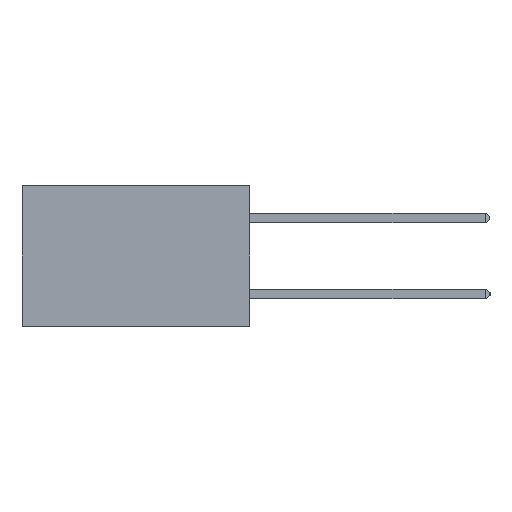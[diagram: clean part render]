
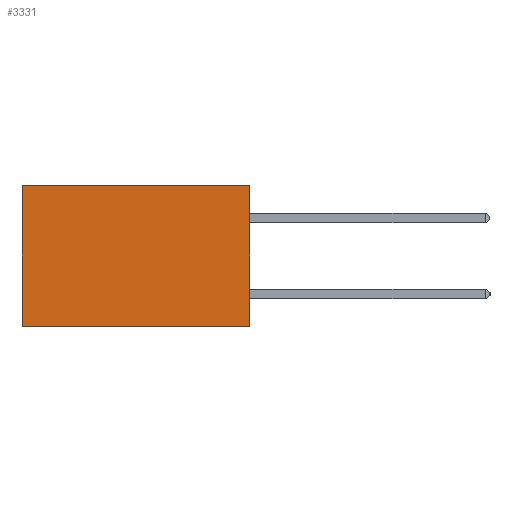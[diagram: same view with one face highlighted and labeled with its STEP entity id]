
A CAD part, left-side view. The second image highlights one B-rep face of the part: STEP entity #3331.
In plain terms, the highlighted planar face has unit normal (-1, 0, 0).
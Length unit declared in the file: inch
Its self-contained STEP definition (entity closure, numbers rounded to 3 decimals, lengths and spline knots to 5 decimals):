
#175 = VECTOR ( 'NONE', #521, 39.37008 ) ;
#521 = DIRECTION ( 'NONE',  ( 0., 1., 0. ) ) ;
#916 = EDGE_CURVE ( 'NONE', #8015, #15367, #3293, .T. ) ;
#978 = LINE ( 'NONE', #11055, #4941 ) ;
#2094 = CARTESIAN_POINT ( 'NONE',  ( 0.2875, 0., 0. ) ) ;
#3293 = LINE ( 'NONE', #18927, #20393 ) ;
#3331 = ADVANCED_FACE ( 'NONE', ( #19078 ), #16907, .F. ) ;
#3595 = EDGE_CURVE ( 'NONE', #15367, #18838, #9083, .T. ) ;
#4389 = DIRECTION ( 'NONE',  ( 0., 1., 0. ) ) ;
#4941 = VECTOR ( 'NONE', #12691, 39.37008 ) ;
#7116 = CARTESIAN_POINT ( 'NONE',  ( 0.2875, 0., 0. ) ) ;
#8015 = VERTEX_POINT ( 'NONE', #2094 ) ;
#9083 = LINE ( 'NONE', #15950, #13371 ) ;
#10368 = EDGE_LOOP ( 'NONE', ( #21266, #17942, #12976, #20442 ) ) ;
#10464 = DIRECTION ( 'NONE',  ( 0., 0., -1. ) ) ;
#11055 = CARTESIAN_POINT ( 'NONE',  ( 0.2875, 0.6, 0. ) ) ;
#11989 = CARTESIAN_POINT ( 'NONE',  ( 0.2875, 0., -0.37 ) ) ;
#12459 = VERTEX_POINT ( 'NONE', #13871 ) ;
#12691 = DIRECTION ( 'NONE',  ( 0., 0., -1. ) ) ;
#12694 = CARTESIAN_POINT ( 'NONE',  ( 0.2875, 0.6, -0.37 ) ) ;
#12976 = ORIENTED_EDGE ( 'NONE', *, *, #916, .F. ) ;
#13371 = VECTOR ( 'NONE', #4389, 39.37008 ) ;
#13849 = CARTESIAN_POINT ( 'NONE',  ( 0.2875, 0., 0. ) ) ;
#13871 = CARTESIAN_POINT ( 'NONE',  ( 0.2875, 0.6, 0. ) ) ;
#15367 = VERTEX_POINT ( 'NONE', #11989 ) ;
#15950 = CARTESIAN_POINT ( 'NONE',  ( 0.2875, 0., -0.37 ) ) ;
#16742 = EDGE_CURVE ( 'NONE', #8015, #12459, #17345, .T. ) ;
#16907 = PLANE ( 'NONE',  #19900 ) ;
#17345 = LINE ( 'NONE', #13849, #175 ) ;
#17942 = ORIENTED_EDGE ( 'NONE', *, *, #3595, .F. ) ;
#18838 = VERTEX_POINT ( 'NONE', #12694 ) ;
#18927 = CARTESIAN_POINT ( 'NONE',  ( 0.2875, 0., 0. ) ) ;
#19078 = FACE_OUTER_BOUND ( 'NONE', #10368, .T. ) ;
#19900 = AXIS2_PLACEMENT_3D ( 'NONE', #7116, #20269, #10464 ) ;
#20269 = DIRECTION ( 'NONE',  ( 1., 0., 0. ) ) ;
#20388 = EDGE_CURVE ( 'NONE', #12459, #18838, #978, .T. ) ;
#20393 = VECTOR ( 'NONE', #20552, 39.37008 ) ;
#20442 = ORIENTED_EDGE ( 'NONE', *, *, #16742, .T. ) ;
#20552 = DIRECTION ( 'NONE',  ( 0., 0., -1. ) ) ;
#21266 = ORIENTED_EDGE ( 'NONE', *, *, #20388, .T. ) ;
